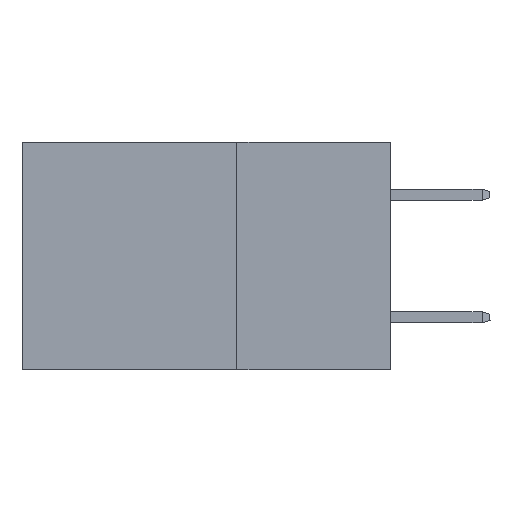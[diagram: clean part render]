
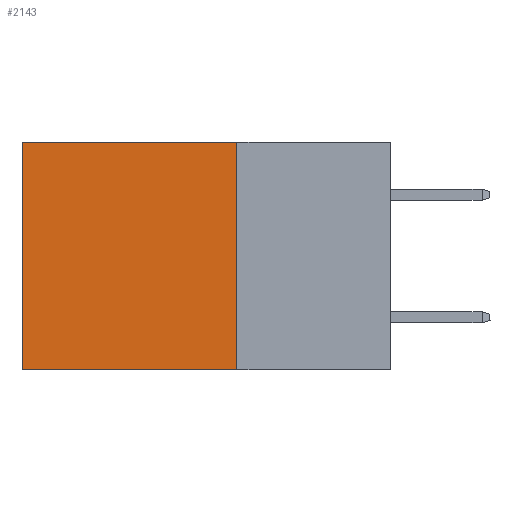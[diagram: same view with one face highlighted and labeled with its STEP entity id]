
A CAD part, left-side view. The second image highlights one B-rep face of the part: STEP entity #2143.
In plain terms, the highlighted planar face has unit normal (-1, 0, 0).
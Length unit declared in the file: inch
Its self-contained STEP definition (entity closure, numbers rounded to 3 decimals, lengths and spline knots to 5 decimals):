
#336 = VECTOR ( 'NONE', #1787, 39.37008 ) ;
#374 = VERTEX_POINT ( 'NONE', #4078 ) ;
#1276 = VERTEX_POINT ( 'NONE', #6264 ) ;
#1787 = DIRECTION ( 'NONE',  ( 0., 1., 0. ) ) ;
#2143 = ADVANCED_FACE ( 'NONE', ( #9464 ), #13015, .F. ) ;
#2260 = AXIS2_PLACEMENT_3D ( 'NONE', #2566, #14637, #13361 ) ;
#2566 = CARTESIAN_POINT ( 'NONE',  ( 0.2875, 0.25, 0. ) ) ;
#2767 = LINE ( 'NONE', #12108, #15527 ) ;
#2963 = CARTESIAN_POINT ( 'NONE',  ( 0.2875, 0.25, 0. ) ) ;
#3902 = LINE ( 'NONE', #2963, #336 ) ;
#4041 = EDGE_CURVE ( 'NONE', #1276, #374, #12858, .T. ) ;
#4078 = CARTESIAN_POINT ( 'NONE',  ( 0.2875, 0.25, -0.37 ) ) ;
#4476 = ORIENTED_EDGE ( 'NONE', *, *, #4041, .F. ) ;
#4979 = CARTESIAN_POINT ( 'NONE',  ( 0.2875, 0.6, 0. ) ) ;
#4993 = ORIENTED_EDGE ( 'NONE', *, *, #5184, .F. ) ;
#5018 = CARTESIAN_POINT ( 'NONE',  ( 0.2875, 0.6, 0. ) ) ;
#5184 = EDGE_CURVE ( 'NONE', #374, #13488, #2767, .T. ) ;
#5320 = VECTOR ( 'NONE', #16588, 39.37008 ) ;
#6081 = EDGE_LOOP ( 'NONE', ( #12702, #4993, #4476, #6499 ) ) ;
#6264 = CARTESIAN_POINT ( 'NONE',  ( 0.2875, 0.25, 0. ) ) ;
#6499 = ORIENTED_EDGE ( 'NONE', *, *, #8899, .T. ) ;
#7694 = DIRECTION ( 'NONE',  ( 0., 0., -1. ) ) ;
#8063 = DIRECTION ( 'NONE',  ( 0., 1., 0. ) ) ;
#8899 = EDGE_CURVE ( 'NONE', #1276, #12745, #3902, .T. ) ;
#9043 = CARTESIAN_POINT ( 'NONE',  ( 0.2875, 0.6, -0.37 ) ) ;
#9464 = FACE_OUTER_BOUND ( 'NONE', #6081, .T. ) ;
#11067 = VECTOR ( 'NONE', #7694, 39.37008 ) ;
#12108 = CARTESIAN_POINT ( 'NONE',  ( 0.2875, 0.25, -0.37 ) ) ;
#12702 = ORIENTED_EDGE ( 'NONE', *, *, #16375, .T. ) ;
#12745 = VERTEX_POINT ( 'NONE', #4979 ) ;
#12858 = LINE ( 'NONE', #16473, #5320 ) ;
#13015 = PLANE ( 'NONE',  #2260 ) ;
#13361 = DIRECTION ( 'NONE',  ( 0., 0., -1. ) ) ;
#13488 = VERTEX_POINT ( 'NONE', #9043 ) ;
#13994 = LINE ( 'NONE', #5018, #11067 ) ;
#14637 = DIRECTION ( 'NONE',  ( 1., 0., 0. ) ) ;
#15527 = VECTOR ( 'NONE', #8063, 39.37008 ) ;
#16375 = EDGE_CURVE ( 'NONE', #12745, #13488, #13994, .T. ) ;
#16473 = CARTESIAN_POINT ( 'NONE',  ( 0.2875, 0.25, 0. ) ) ;
#16588 = DIRECTION ( 'NONE',  ( 0., 0., -1. ) ) ;
